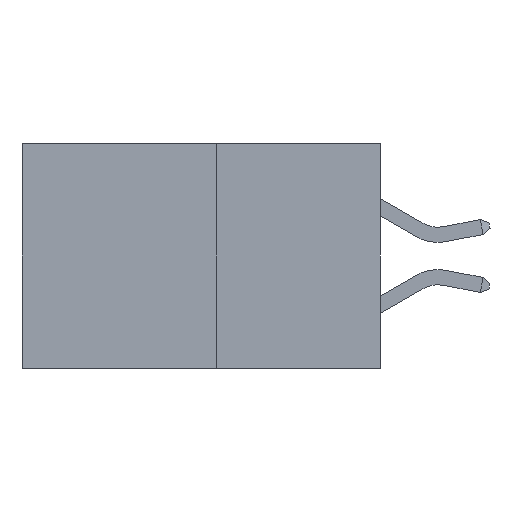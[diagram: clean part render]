
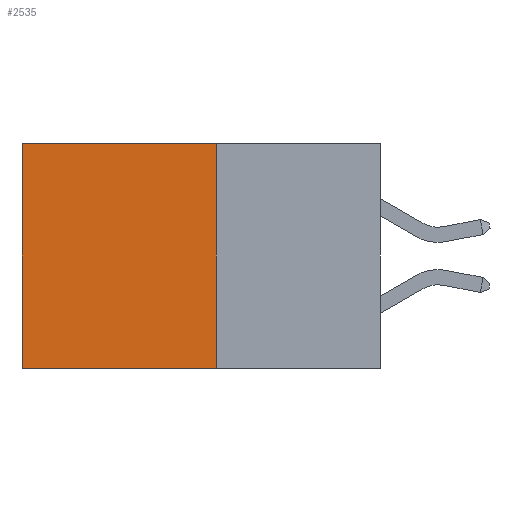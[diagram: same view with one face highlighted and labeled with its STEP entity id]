
A CAD part, left-side view. The second image highlights one B-rep face of the part: STEP entity #2535.
In plain terms, the highlighted planar face has unit normal (-1, 0, 0).
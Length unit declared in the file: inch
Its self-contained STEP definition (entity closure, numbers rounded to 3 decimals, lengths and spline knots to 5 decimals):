
#118 = CARTESIAN_POINT ( 'NONE',  ( 0.277, 0.59, 0. ) ) ;
#1647 = VERTEX_POINT ( 'NONE', #3916 ) ;
#2535 = ADVANCED_FACE ( 'NONE', ( #9662 ), #2943, .F. ) ;
#2865 = VECTOR ( 'NONE', #12997, 39.37008 ) ;
#2881 = AXIS2_PLACEMENT_3D ( 'NONE', #14205, #13290, #11022 ) ;
#2943 = PLANE ( 'NONE',  #2881 ) ;
#3702 = VECTOR ( 'NONE', #11432, 39.37008 ) ;
#3733 = CARTESIAN_POINT ( 'NONE',  ( 0.277, 0.59, -0.37 ) ) ;
#3916 = CARTESIAN_POINT ( 'NONE',  ( 0.277, 0.27, -0.37 ) ) ;
#4039 = CARTESIAN_POINT ( 'NONE',  ( 0.277, 0.27, -0.37 ) ) ;
#4196 = EDGE_CURVE ( 'NONE', #9982, #9761, #4752, .T. ) ;
#4442 = ORIENTED_EDGE ( 'NONE', *, *, #6485, .F. ) ;
#4752 = LINE ( 'NONE', #9347, #16592 ) ;
#5964 = DIRECTION ( 'NONE',  ( 0., 1., 0. ) ) ;
#6485 = EDGE_CURVE ( 'NONE', #7200, #1647, #15604, .T. ) ;
#6871 = LINE ( 'NONE', #4039, #2865 ) ;
#7200 = VERTEX_POINT ( 'NONE', #18627 ) ;
#9347 = CARTESIAN_POINT ( 'NONE',  ( 0.277, 0.59, -0.37 ) ) ;
#9662 = FACE_OUTER_BOUND ( 'NONE', #12053, .T. ) ;
#9761 = VERTEX_POINT ( 'NONE', #3733 ) ;
#9982 = VERTEX_POINT ( 'NONE', #118 ) ;
#11022 = DIRECTION ( 'NONE',  ( 0., 0., -1. ) ) ;
#11372 = CARTESIAN_POINT ( 'NONE',  ( 0.277, 0.27, -0.37 ) ) ;
#11432 = DIRECTION ( 'NONE',  ( 0., 0., -1. ) ) ;
#12053 = EDGE_LOOP ( 'NONE', ( #13885, #18119, #4442, #12937 ) ) ;
#12937 = ORIENTED_EDGE ( 'NONE', *, *, #17023, .T. ) ;
#12997 = DIRECTION ( 'NONE',  ( 0., 1., 0. ) ) ;
#13290 = DIRECTION ( 'NONE',  ( 1., 0., 0. ) ) ;
#13885 = ORIENTED_EDGE ( 'NONE', *, *, #4196, .T. ) ;
#14205 = CARTESIAN_POINT ( 'NONE',  ( 0.277, 0.27, -0.37 ) ) ;
#14864 = DIRECTION ( 'NONE',  ( 0., 0., -1. ) ) ;
#14889 = CARTESIAN_POINT ( 'NONE',  ( 0.277, 0.27, 0. ) ) ;
#15604 = LINE ( 'NONE', #11372, #3702 ) ;
#16592 = VECTOR ( 'NONE', #14864, 39.37008 ) ;
#17023 = EDGE_CURVE ( 'NONE', #7200, #9982, #17315, .T. ) ;
#17315 = LINE ( 'NONE', #14889, #17800 ) ;
#17425 = EDGE_CURVE ( 'NONE', #1647, #9761, #6871, .T. ) ;
#17800 = VECTOR ( 'NONE', #5964, 39.37008 ) ;
#18119 = ORIENTED_EDGE ( 'NONE', *, *, #17425, .F. ) ;
#18627 = CARTESIAN_POINT ( 'NONE',  ( 0.277, 0.27, 0. ) ) ;
